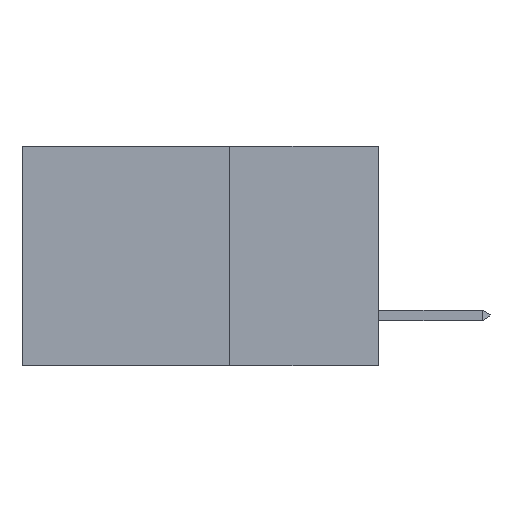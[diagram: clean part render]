
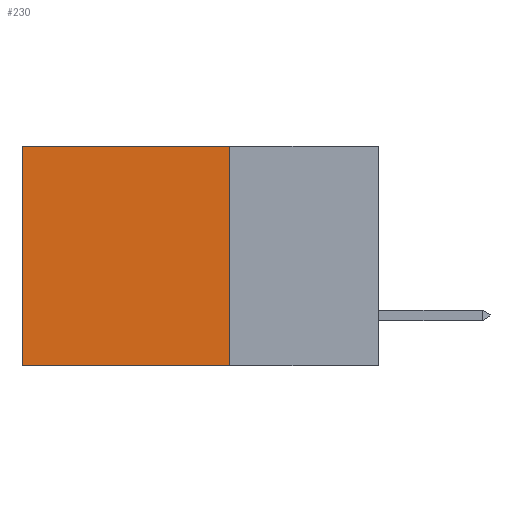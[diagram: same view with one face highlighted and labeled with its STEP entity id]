
A CAD part, left-side view. The second image highlights one B-rep face of the part: STEP entity #230.
In plain terms, the highlighted planar face has unit normal (-1, 0, 0).
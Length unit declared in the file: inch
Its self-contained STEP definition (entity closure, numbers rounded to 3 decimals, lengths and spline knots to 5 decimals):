
#65 = FACE_OUTER_BOUND ( 'NONE', #14730, .T. ) ;
#230 = ADVANCED_FACE ( 'NONE', ( #65 ), #3167, .F. ) ;
#416 = CARTESIAN_POINT ( 'NONE',  ( 0.2615, 0.25, -0.37 ) ) ;
#474 = DIRECTION ( 'NONE',  ( 0., 0., -1. ) ) ;
#920 = ORIENTED_EDGE ( 'NONE', *, *, #14331, .F. ) ;
#1106 = VECTOR ( 'NONE', #474, 39.37008 ) ;
#2346 = EDGE_CURVE ( 'NONE', #11336, #3574, #10176, .T. ) ;
#2658 = CARTESIAN_POINT ( 'NONE',  ( 0.2615, 0.25, 0. ) ) ;
#2989 = LINE ( 'NONE', #3164, #6792 ) ;
#3164 = CARTESIAN_POINT ( 'NONE',  ( 0.2615, 0.25, -0.37 ) ) ;
#3167 = PLANE ( 'NONE',  #15921 ) ;
#3297 = CARTESIAN_POINT ( 'NONE',  ( 0.2615, 0.25, -0.37 ) ) ;
#3359 = VECTOR ( 'NONE', #17325, 39.37008 ) ;
#3574 = VERTEX_POINT ( 'NONE', #12857 ) ;
#4881 = LINE ( 'NONE', #3297, #1106 ) ;
#5337 = EDGE_CURVE ( 'NONE', #12899, #6661, #2989, .T. ) ;
#5845 = CARTESIAN_POINT ( 'NONE',  ( 0.2615, 0.6, -0.37 ) ) ;
#5914 = ORIENTED_EDGE ( 'NONE', *, *, #5337, .F. ) ;
#6661 = VERTEX_POINT ( 'NONE', #14612 ) ;
#6792 = VECTOR ( 'NONE', #11435, 39.37008 ) ;
#7962 = ORIENTED_EDGE ( 'NONE', *, *, #2346, .T. ) ;
#8496 = VECTOR ( 'NONE', #12911, 39.37008 ) ;
#9909 = EDGE_CURVE ( 'NONE', #3574, #6661, #12999, .T. ) ;
#10176 = LINE ( 'NONE', #14517, #8496 ) ;
#11336 = VERTEX_POINT ( 'NONE', #2658 ) ;
#11401 = ORIENTED_EDGE ( 'NONE', *, *, #9909, .T. ) ;
#11435 = DIRECTION ( 'NONE',  ( 0., 1., 0. ) ) ;
#11438 = CARTESIAN_POINT ( 'NONE',  ( 0.2615, 0.25, -0.37 ) ) ;
#11529 = DIRECTION ( 'NONE',  ( 1., 0., 0. ) ) ;
#12857 = CARTESIAN_POINT ( 'NONE',  ( 0.2615, 0.6, 0. ) ) ;
#12899 = VERTEX_POINT ( 'NONE', #416 ) ;
#12911 = DIRECTION ( 'NONE',  ( 0., 1., 0. ) ) ;
#12999 = LINE ( 'NONE', #5845, #3359 ) ;
#14331 = EDGE_CURVE ( 'NONE', #11336, #12899, #4881, .T. ) ;
#14517 = CARTESIAN_POINT ( 'NONE',  ( 0.2615, 0.25, 0. ) ) ;
#14612 = CARTESIAN_POINT ( 'NONE',  ( 0.2615, 0.6, -0.37 ) ) ;
#14630 = DIRECTION ( 'NONE',  ( 0., 0., -1. ) ) ;
#14730 = EDGE_LOOP ( 'NONE', ( #11401, #5914, #920, #7962 ) ) ;
#15921 = AXIS2_PLACEMENT_3D ( 'NONE', #11438, #11529, #14630 ) ;
#17325 = DIRECTION ( 'NONE',  ( 0., 0., -1. ) ) ;
